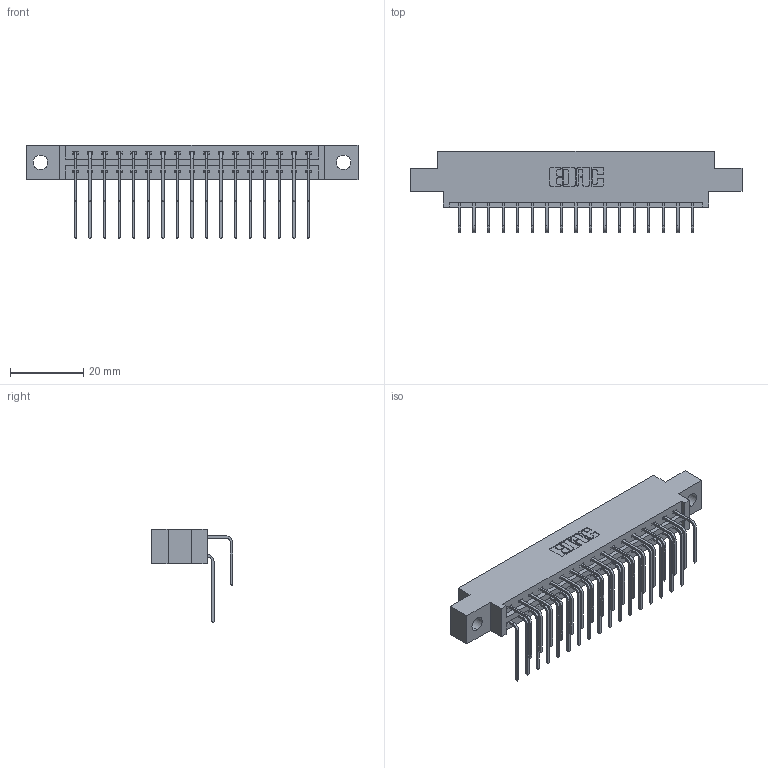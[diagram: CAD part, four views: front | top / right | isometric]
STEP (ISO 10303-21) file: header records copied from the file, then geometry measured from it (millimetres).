
FILE_DESCRIPTION (( 'STEP AP203' ), '1' );
FILE_NAME ('337-034-558-804.STEP', '2018-08-07T19:16:49', ( '' ), ( '' ), 'SwSTEP 2.0', 'SolidWorks 2016', '' );
FILE_SCHEMA (( 'CONFIG_CONTROL_DESIGN' ));
Length unit declared in the file: inch
Products named in the file (4): 345-292-001_558 559 Tail - 1; 337 Part_0.170 Offset - 0.156 Dia-TH; 345-292-001_558 Tail - 2; 337-034-558-804
Assembly tree (35 placements, depth 2):
  337-034-558-804
    337 Part_0.170 Offset - 0.156 Dia-TH
    345-292-001_558 559 Tail - 1  x17
    345-292-001_558 Tail - 2  x17
Bounding box: 90.37 x 22.17 x 25.53 mm (x, y, z)
Volume: 9182.2 mm3; surface area: 11027.8 mm2
Topology: 35 solids, 35 shells, 2022 faces, 6001 edges, 3954 vertices
Faces by surface type: plane 1434, cylinder 588
Entity records: 18333 total; most frequent: CARTESIAN_POINT 3157, ORIENTED_EDGE 3042, DIRECTION 2713, EDGE_CURVE 1521, LINE 1353, VECTOR 1353, VERTEX_POINT 1010, AXIS2_PLACEMENT_3D 680
